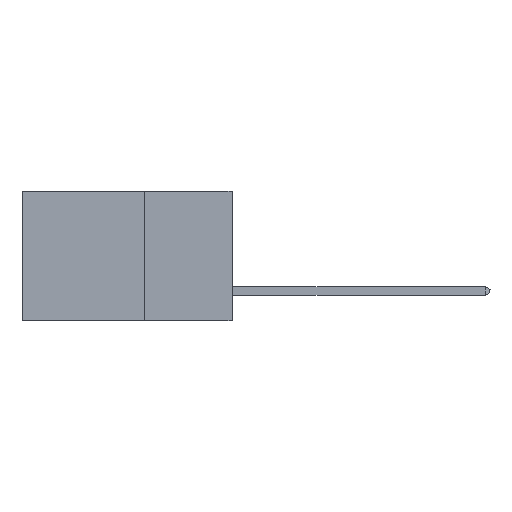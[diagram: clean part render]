
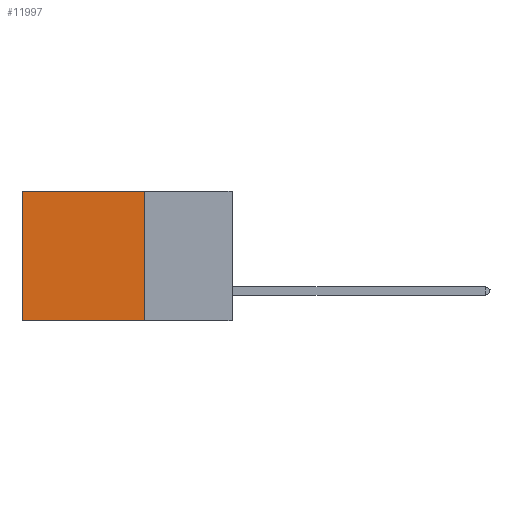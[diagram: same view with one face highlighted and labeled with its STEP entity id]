
A CAD part, left-side view. The second image highlights one B-rep face of the part: STEP entity #11997.
In plain terms, the highlighted planar face has unit normal (-1, 0, 0).
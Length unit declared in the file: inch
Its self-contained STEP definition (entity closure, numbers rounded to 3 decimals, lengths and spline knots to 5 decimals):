
#547 = CARTESIAN_POINT ( 'NONE',  ( 0.2875, 0.25, 0. ) ) ;
#3040 = CARTESIAN_POINT ( 'NONE',  ( 0.2875, 0.25, -0.37 ) ) ;
#4292 = VECTOR ( 'NONE', #44905, 39.37008 ) ;
#4339 = CARTESIAN_POINT ( 'NONE',  ( 0.2875, 0.6, 0. ) ) ;
#6793 = VERTEX_POINT ( 'NONE', #30537 ) ;
#10475 = VECTOR ( 'NONE', #45673, 39.37008 ) ;
#10718 = EDGE_CURVE ( 'NONE', #32575, #28431, #43297, .T. ) ;
#11997 = ADVANCED_FACE ( 'NONE', ( #27214 ), #18668, .F. ) ;
#13411 = CARTESIAN_POINT ( 'NONE',  ( 0.2875, 0.6, -0.37 ) ) ;
#13487 = EDGE_CURVE ( 'NONE', #22161, #28431, #18714, .T. ) ;
#14148 = DIRECTION ( 'NONE',  ( 0., 0., -1. ) ) ;
#16902 = ORIENTED_EDGE ( 'NONE', *, *, #37197, .F. ) ;
#18018 = DIRECTION ( 'NONE',  ( 0., 0., -1. ) ) ;
#18668 = PLANE ( 'NONE',  #43516 ) ;
#18714 = LINE ( 'NONE', #3040, #41781 ) ;
#21415 = CARTESIAN_POINT ( 'NONE',  ( 0.2875, 0.25, 0. ) ) ;
#21706 = EDGE_CURVE ( 'NONE', #6793, #32575, #41774, .T. ) ;
#22161 = VERTEX_POINT ( 'NONE', #33417 ) ;
#25464 = DIRECTION ( 'NONE',  ( 0., 1., 0. ) ) ;
#25928 = CARTESIAN_POINT ( 'NONE',  ( 0.2875, 0.25, 0. ) ) ;
#27214 = FACE_OUTER_BOUND ( 'NONE', #37632, .T. ) ;
#28431 = VERTEX_POINT ( 'NONE', #13411 ) ;
#28538 = ORIENTED_EDGE ( 'NONE', *, *, #13487, .F. ) ;
#30537 = CARTESIAN_POINT ( 'NONE',  ( 0.2875, 0.25, 0. ) ) ;
#32575 = VERTEX_POINT ( 'NONE', #4339 ) ;
#33417 = CARTESIAN_POINT ( 'NONE',  ( 0.2875, 0.25, -0.37 ) ) ;
#33429 = DIRECTION ( 'NONE',  ( 1., 0., 0. ) ) ;
#33808 = CARTESIAN_POINT ( 'NONE',  ( 0.2875, 0.6, 0. ) ) ;
#35226 = ORIENTED_EDGE ( 'NONE', *, *, #21706, .T. ) ;
#37197 = EDGE_CURVE ( 'NONE', #6793, #22161, #42716, .T. ) ;
#37632 = EDGE_LOOP ( 'NONE', ( #41858, #28538, #16902, #35226 ) ) ;
#41774 = LINE ( 'NONE', #547, #10475 ) ;
#41781 = VECTOR ( 'NONE', #25464, 39.37008 ) ;
#41858 = ORIENTED_EDGE ( 'NONE', *, *, #10718, .T. ) ;
#42716 = LINE ( 'NONE', #21415, #43939 ) ;
#43297 = LINE ( 'NONE', #33808, #4292 ) ;
#43516 = AXIS2_PLACEMENT_3D ( 'NONE', #25928, #33429, #18018 ) ;
#43939 = VECTOR ( 'NONE', #14148, 39.37008 ) ;
#44905 = DIRECTION ( 'NONE',  ( 0., 0., -1. ) ) ;
#45673 = DIRECTION ( 'NONE',  ( 0., 1., 0. ) ) ;
